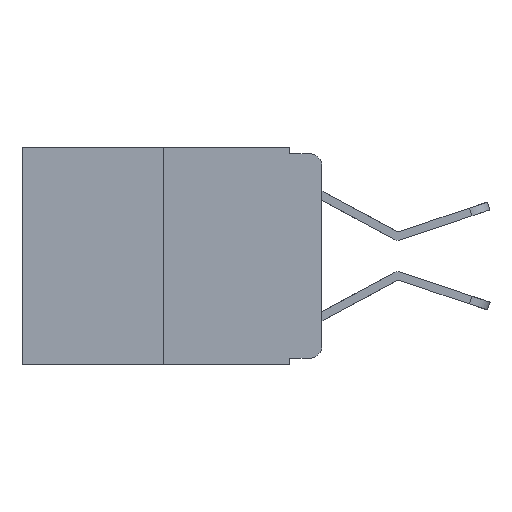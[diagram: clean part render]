
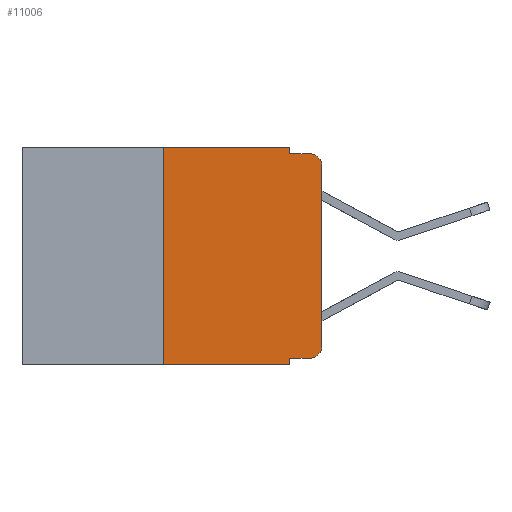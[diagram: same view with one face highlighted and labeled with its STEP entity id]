
A CAD part, left-side view. The second image highlights one B-rep face of the part: STEP entity #11006.
In plain terms, the highlighted planar face has unit normal (-1, 0, 0).
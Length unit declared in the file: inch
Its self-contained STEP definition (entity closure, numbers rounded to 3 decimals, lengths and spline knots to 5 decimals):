
#243 = CARTESIAN_POINT ( 'NONE',  ( 0., 0.051, 0. ) ) ;
#316 = FACE_OUTER_BOUND ( 'NONE', #10099, .T. ) ;
#406 = LINE ( 'NONE', #12085, #10326 ) ;
#417 = VERTEX_POINT ( 'NONE', #243 ) ;
#480 = LINE ( 'NONE', #9477, #12370 ) ;
#938 = CARTESIAN_POINT ( 'NONE',  ( 0., 0.051, 0. ) ) ;
#969 = VERTEX_POINT ( 'NONE', #2184 ) ;
#1249 = ORIENTED_EDGE ( 'NONE', *, *, #8025, .T. ) ;
#1323 = DIRECTION ( 'NONE',  ( 0., -1., 0. ) ) ;
#1732 = DIRECTION ( 'NONE',  ( 0., -1., 0. ) ) ;
#2184 = CARTESIAN_POINT ( 'NONE',  ( 0., 0.25, 0. ) ) ;
#2567 = CARTESIAN_POINT ( 'NONE',  ( 0., 0.051, -0.333 ) ) ;
#2772 = EDGE_CURVE ( 'NONE', #969, #417, #6263, .T. ) ;
#2944 = CARTESIAN_POINT ( 'NONE',  ( 0., 0.02, -0.333 ) ) ;
#2949 = VERTEX_POINT ( 'NONE', #2944 ) ;
#3103 = AXIS2_PLACEMENT_3D ( 'NONE', #8132, #14406, #14489 ) ;
#3105 = DIRECTION ( 'NONE',  ( 0., 0., -1. ) ) ;
#3192 = DIRECTION ( 'NONE',  ( -1., 0., 0. ) ) ;
#3237 = DIRECTION ( 'NONE',  ( 0., 0., -1. ) ) ;
#3377 = EDGE_CURVE ( 'NONE', #417, #13415, #406, .T. ) ;
#3730 = VERTEX_POINT ( 'NONE', #13892 ) ;
#3768 = CARTESIAN_POINT ( 'NONE',  ( 0., 0.473, 0. ) ) ;
#3796 = ORIENTED_EDGE ( 'NONE', *, *, #16321, .T. ) ;
#3895 = CIRCLE ( 'NONE', #3103, 0.02 ) ;
#4045 = EDGE_CURVE ( 'NONE', #13415, #11030, #7444, .T. ) ;
#4134 = CARTESIAN_POINT ( 'NONE',  ( 0., 0., -0.313 ) ) ;
#4318 = AXIS2_PLACEMENT_3D ( 'NONE', #15559, #10628, #15046 ) ;
#4326 = DIRECTION ( 'NONE',  ( 0., 0., -1. ) ) ;
#4358 = ORIENTED_EDGE ( 'NONE', *, *, #4045, .F. ) ;
#6263 = LINE ( 'NONE', #3768, #15372 ) ;
#6539 = LINE ( 'NONE', #2567, #15456 ) ;
#6789 = CARTESIAN_POINT ( 'NONE',  ( 0., 0.25, 0. ) ) ;
#7009 = LINE ( 'NONE', #938, #10692 ) ;
#7086 = CARTESIAN_POINT ( 'NONE',  ( 0., 0.02, -0.03 ) ) ;
#7444 = LINE ( 'NONE', #11134, #9566 ) ;
#7665 = CARTESIAN_POINT ( 'NONE',  ( 0., 0.051, -0.01 ) ) ;
#8025 = EDGE_CURVE ( 'NONE', #2949, #13527, #3895, .T. ) ;
#8054 = ORIENTED_EDGE ( 'NONE', *, *, #10308, .F. ) ;
#8132 = CARTESIAN_POINT ( 'NONE',  ( 0., 0.02, -0.313 ) ) ;
#8319 = VECTOR ( 'NONE', #10795, 39.37008 ) ;
#8357 = VERTEX_POINT ( 'NONE', #8806 ) ;
#8486 = AXIS2_PLACEMENT_3D ( 'NONE', #7086, #3192, #4326 ) ;
#8806 = CARTESIAN_POINT ( 'NONE',  ( 0., 0.051, -0.333 ) ) ;
#8970 = EDGE_CURVE ( 'NONE', #15081, #11030, #10891, .T. ) ;
#9462 = CARTESIAN_POINT ( 'NONE',  ( 0., 0., -0.03 ) ) ;
#9477 = CARTESIAN_POINT ( 'NONE',  ( 0., 0.473, -0.343 ) ) ;
#9566 = VECTOR ( 'NONE', #9928, 39.37008 ) ;
#9656 = EDGE_CURVE ( 'NONE', #8357, #2949, #6539, .T. ) ;
#9928 = DIRECTION ( 'NONE',  ( 0., -1., 0. ) ) ;
#10099 = EDGE_LOOP ( 'NONE', ( #3796, #15272, #4358, #10811, #10752, #15612, #14343, #8054, #10254, #1249 ) ) ;
#10254 = ORIENTED_EDGE ( 'NONE', *, *, #9656, .T. ) ;
#10308 = EDGE_CURVE ( 'NONE', #8357, #15351, #7009, .T. ) ;
#10326 = VECTOR ( 'NONE', #3237, 39.37008 ) ;
#10378 = CARTESIAN_POINT ( 'NONE',  ( 0., 0., 0. ) ) ;
#10466 = PLANE ( 'NONE',  #4318 ) ;
#10628 = DIRECTION ( 'NONE',  ( 1., 0., 0. ) ) ;
#10692 = VECTOR ( 'NONE', #3105, 39.37008 ) ;
#10752 = ORIENTED_EDGE ( 'NONE', *, *, #2772, .F. ) ;
#10795 = DIRECTION ( 'NONE',  ( 0., 0., 1. ) ) ;
#10811 = ORIENTED_EDGE ( 'NONE', *, *, #3377, .F. ) ;
#10891 = CIRCLE ( 'NONE', #8486, 0.02 ) ;
#11006 = ADVANCED_FACE ( 'NONE', ( #316 ), #10466, .F. ) ;
#11030 = VERTEX_POINT ( 'NONE', #13704 ) ;
#11134 = CARTESIAN_POINT ( 'NONE',  ( 0., 0.051, -0.01 ) ) ;
#11384 = DIRECTION ( 'NONE',  ( 0., -1., 0. ) ) ;
#11891 = LINE ( 'NONE', #10378, #13412 ) ;
#11983 = DIRECTION ( 'NONE',  ( 0., 0., 1. ) ) ;
#12085 = CARTESIAN_POINT ( 'NONE',  ( 0., 0.051, 0. ) ) ;
#12248 = EDGE_CURVE ( 'NONE', #3730, #969, #13227, .T. ) ;
#12301 = EDGE_CURVE ( 'NONE', #3730, #15351, #480, .T. ) ;
#12370 = VECTOR ( 'NONE', #1732, 39.37008 ) ;
#13227 = LINE ( 'NONE', #6789, #8319 ) ;
#13412 = VECTOR ( 'NONE', #11983, 39.37008 ) ;
#13415 = VERTEX_POINT ( 'NONE', #7665 ) ;
#13527 = VERTEX_POINT ( 'NONE', #4134 ) ;
#13704 = CARTESIAN_POINT ( 'NONE',  ( 0., 0.02, -0.01 ) ) ;
#13892 = CARTESIAN_POINT ( 'NONE',  ( 0., 0.25, -0.343 ) ) ;
#14343 = ORIENTED_EDGE ( 'NONE', *, *, #12301, .T. ) ;
#14406 = DIRECTION ( 'NONE',  ( -1., 0., 0. ) ) ;
#14489 = DIRECTION ( 'NONE',  ( 0., 0., -1. ) ) ;
#15046 = DIRECTION ( 'NONE',  ( 0., 0., -1. ) ) ;
#15081 = VERTEX_POINT ( 'NONE', #9462 ) ;
#15122 = CARTESIAN_POINT ( 'NONE',  ( 0., 0.051, -0.343 ) ) ;
#15272 = ORIENTED_EDGE ( 'NONE', *, *, #8970, .T. ) ;
#15351 = VERTEX_POINT ( 'NONE', #15122 ) ;
#15372 = VECTOR ( 'NONE', #11384, 39.37008 ) ;
#15456 = VECTOR ( 'NONE', #1323, 39.37008 ) ;
#15559 = CARTESIAN_POINT ( 'NONE',  ( 0., 0.473, 0. ) ) ;
#15612 = ORIENTED_EDGE ( 'NONE', *, *, #12248, .F. ) ;
#16321 = EDGE_CURVE ( 'NONE', #13527, #15081, #11891, .T. ) ;
